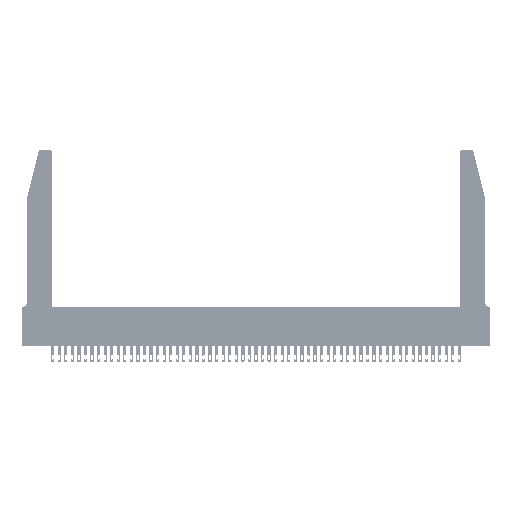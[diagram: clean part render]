
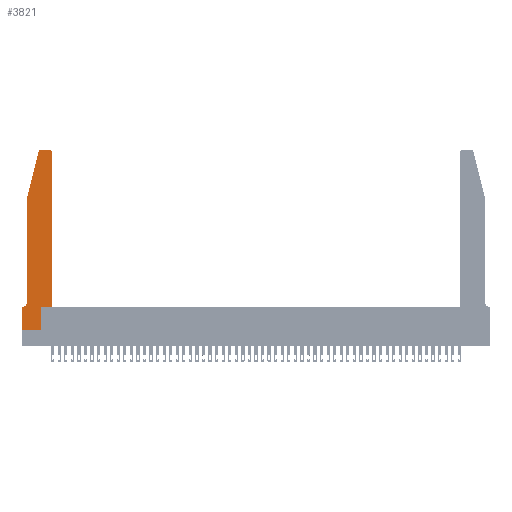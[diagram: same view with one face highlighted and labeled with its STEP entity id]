
A CAD part, top view. The second image highlights one B-rep face of the part: STEP entity #3821.
In plain terms, the highlighted planar face has unit normal (0, 0, 1).
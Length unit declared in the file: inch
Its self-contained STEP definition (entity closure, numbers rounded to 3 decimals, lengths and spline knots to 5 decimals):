
#220 = EDGE_CURVE ( 'NONE', #26783, #27780, #22821, .T. ) ;
#998 = CARTESIAN_POINT ( 'NONE',  ( 0.4505, 0.35, 0.37 ) ) ;
#1057 = EDGE_CURVE ( 'NONE', #46100, #28939, #23431, .T. ) ;
#1085 = VERTEX_POINT ( 'NONE', #23866 ) ;
#2592 = CARTESIAN_POINT ( 'NONE',  ( 0., 0.35, 0.37 ) ) ;
#3109 = DIRECTION ( 'NONE',  ( -0.239, -0.971, 0. ) ) ;
#3821 = ADVANCED_FACE ( 'NONE', ( #13299 ), #21908, .T. ) ;
#4509 = EDGE_CURVE ( 'NONE', #28374, #39760, #44208, .T. ) ;
#4977 = DIRECTION ( 'NONE',  ( 0., 1., 0. ) ) ;
#5112 = VERTEX_POINT ( 'NONE', #32635 ) ;
#6354 = VERTEX_POINT ( 'NONE', #34230 ) ;
#6897 = EDGE_CURVE ( 'NONE', #25672, #26783, #39612, .T. ) ;
#7028 = EDGE_CURVE ( 'NONE', #1085, #46100, #27404, .T. ) ;
#7814 = DIRECTION ( 'NONE',  ( 0., -1., 0. ) ) ;
#8128 = DIRECTION ( 'NONE',  ( -1., 0., 0. ) ) ;
#8252 = ORIENTED_EDGE ( 'NONE', *, *, #4509, .T. ) ;
#8278 = CARTESIAN_POINT ( 'NONE',  ( 0.0755, 2., 0.37 ) ) ;
#10289 = CARTESIAN_POINT ( 'NONE',  ( 0., 0.35, 0.37 ) ) ;
#10340 = CARTESIAN_POINT ( 'NONE',  ( 0.2865, 0.35, 0.37 ) ) ;
#10620 = CARTESIAN_POINT ( 'NONE',  ( 0.0755, 0.42, 0.37 ) ) ;
#12246 = CARTESIAN_POINT ( 'NONE',  ( 0.0055, 0.42, 0.37 ) ) ;
#12318 = CARTESIAN_POINT ( 'NONE',  ( 0.4205, 2.72, 0.37 ) ) ;
#12788 = VECTOR ( 'NONE', #3109, 39.37008 ) ;
#13299 = FACE_OUTER_BOUND ( 'NONE', #31462, .T. ) ;
#14311 = DIRECTION ( 'NONE',  ( -1., 0., 0. ) ) ;
#16272 = DIRECTION ( 'NONE',  ( 0., 0., 1. ) ) ;
#16526 = VECTOR ( 'NONE', #48999, 39.37008 ) ;
#16605 = CARTESIAN_POINT ( 'NONE',  ( 0., 0., 0.37 ) ) ;
#16889 = VECTOR ( 'NONE', #35696, 39.37008 ) ;
#18139 = ORIENTED_EDGE ( 'NONE', *, *, #7028, .T. ) ;
#18206 = ORIENTED_EDGE ( 'NONE', *, *, #23813, .T. ) ;
#18840 = CARTESIAN_POINT ( 'NONE',  ( 0.25487, 2.72718, 0.37 ) ) ;
#19865 = EDGE_CURVE ( 'NONE', #34818, #1085, #37081, .T. ) ;
#20961 = ORIENTED_EDGE ( 'NONE', *, *, #220, .T. ) ;
#21037 = DIRECTION ( 'NONE',  ( 1., 0., 0. ) ) ;
#21895 = AXIS2_PLACEMENT_3D ( 'NONE', #12318, #36790, #21037 ) ;
#21908 = PLANE ( 'NONE',  #37344 ) ;
#22610 = DIRECTION ( 'NONE',  ( 0., -1., 0. ) ) ;
#22821 = LINE ( 'NONE', #25040, #16526 ) ;
#23431 = CIRCLE ( 'NONE', #32250, 0.03 ) ;
#23733 = CARTESIAN_POINT ( 'NONE',  ( 0.0055, 0.35, 0.37 ) ) ;
#23813 = EDGE_CURVE ( 'NONE', #27780, #5112, #41073, .T. ) ;
#23866 = CARTESIAN_POINT ( 'NONE',  ( 0.4205, 2.75, 0.37 ) ) ;
#24027 = CARTESIAN_POINT ( 'NONE',  ( 0.284, 2.72, 0.37 ) ) ;
#24239 = ORIENTED_EDGE ( 'NONE', *, *, #48163, .T. ) ;
#25040 = CARTESIAN_POINT ( 'NONE',  ( 0., 0., 0.37 ) ) ;
#25184 = LINE ( 'NONE', #38951, #12788 ) ;
#25672 = VERTEX_POINT ( 'NONE', #2592 ) ;
#25901 = DIRECTION ( 'NONE',  ( 0., 1., 0. ) ) ;
#26783 = VERTEX_POINT ( 'NONE', #16605 ) ;
#26892 = DIRECTION ( 'NONE',  ( 0., 0., 1. ) ) ;
#27404 = LINE ( 'NONE', #34064, #41087 ) ;
#27405 = LINE ( 'NONE', #31038, #16889 ) ;
#27780 = VERTEX_POINT ( 'NONE', #39206 ) ;
#28033 = DIRECTION ( 'NONE',  ( 1., 0., 0. ) ) ;
#28374 = VERTEX_POINT ( 'NONE', #8278 ) ;
#28939 = VERTEX_POINT ( 'NONE', #18840 ) ;
#29830 = CIRCLE ( 'NONE', #51229, 0.07 ) ;
#30172 = DIRECTION ( 'NONE',  ( 1., 0., 0. ) ) ;
#30941 = VECTOR ( 'NONE', #22610, 39.37008 ) ;
#31038 = CARTESIAN_POINT ( 'NONE',  ( 0.0755, 0.35, 0.37 ) ) ;
#31462 = EDGE_LOOP ( 'NONE', ( #18139, #47641, #24239, #8252, #48288, #35584, #42317, #20961, #18206, #38829, #38232, #39391 ) ) ;
#32250 = AXIS2_PLACEMENT_3D ( 'NONE', #24027, #16272, #28033 ) ;
#32542 = VECTOR ( 'NONE', #4977, 39.37008 ) ;
#32635 = CARTESIAN_POINT ( 'NONE',  ( 0.2865, 0.35, 0.37 ) ) ;
#32901 = CARTESIAN_POINT ( 'NONE',  ( 0., 0., 0.37 ) ) ;
#34064 = CARTESIAN_POINT ( 'NONE',  ( 0.2605, 2.75, 0.37 ) ) ;
#34230 = CARTESIAN_POINT ( 'NONE',  ( 0.4505, 0.35, 0.37 ) ) ;
#34818 = VERTEX_POINT ( 'NONE', #42588 ) ;
#35173 = CARTESIAN_POINT ( 'NONE',  ( 0.284, 2.75, 0.37 ) ) ;
#35584 = ORIENTED_EDGE ( 'NONE', *, *, #49959, .T. ) ;
#35696 = DIRECTION ( 'NONE',  ( -1., 0., 0. ) ) ;
#36790 = DIRECTION ( 'NONE',  ( 0., 0., 1. ) ) ;
#37081 = CIRCLE ( 'NONE', #21895, 0.03 ) ;
#37215 = VERTEX_POINT ( 'NONE', #23733 ) ;
#37344 = AXIS2_PLACEMENT_3D ( 'NONE', #10289, #26892, #30172 ) ;
#38232 = ORIENTED_EDGE ( 'NONE', *, *, #48952, .T. ) ;
#38829 = ORIENTED_EDGE ( 'NONE', *, *, #48463, .T. ) ;
#38951 = CARTESIAN_POINT ( 'NONE',  ( 0.0755, 2., 0.37 ) ) ;
#39206 = CARTESIAN_POINT ( 'NONE',  ( 0.2865, 0., 0.37 ) ) ;
#39391 = ORIENTED_EDGE ( 'NONE', *, *, #19865, .T. ) ;
#39612 = LINE ( 'NONE', #32901, #30941 ) ;
#39760 = VERTEX_POINT ( 'NONE', #10620 ) ;
#39984 = DIRECTION ( 'NONE',  ( 0., 0., -1. ) ) ;
#41073 = LINE ( 'NONE', #10340, #50370 ) ;
#41087 = VECTOR ( 'NONE', #14311, 39.37008 ) ;
#41505 = CARTESIAN_POINT ( 'NONE',  ( 0.4505, 0.35, 0.37 ) ) ;
#42317 = ORIENTED_EDGE ( 'NONE', *, *, #6897, .T. ) ;
#42461 = EDGE_CURVE ( 'NONE', #39760, #37215, #29830, .T. ) ;
#42588 = CARTESIAN_POINT ( 'NONE',  ( 0.4505, 2.72, 0.37 ) ) ;
#43116 = LINE ( 'NONE', #998, #32542 ) ;
#43498 = CARTESIAN_POINT ( 'NONE',  ( 0.0755, 2., 0.37 ) ) ;
#44208 = LINE ( 'NONE', #43498, #47944 ) ;
#45125 = DIRECTION ( 'NONE',  ( 1., 0., 0. ) ) ;
#45662 = LINE ( 'NONE', #41505, #49987 ) ;
#46100 = VERTEX_POINT ( 'NONE', #35173 ) ;
#47641 = ORIENTED_EDGE ( 'NONE', *, *, #1057, .T. ) ;
#47944 = VECTOR ( 'NONE', #7814, 39.37008 ) ;
#48163 = EDGE_CURVE ( 'NONE', #28939, #28374, #25184, .T. ) ;
#48288 = ORIENTED_EDGE ( 'NONE', *, *, #42461, .T. ) ;
#48463 = EDGE_CURVE ( 'NONE', #5112, #6354, #45662, .T. ) ;
#48952 = EDGE_CURVE ( 'NONE', #6354, #34818, #43116, .T. ) ;
#48999 = DIRECTION ( 'NONE',  ( 1., 0., 0. ) ) ;
#49959 = EDGE_CURVE ( 'NONE', #37215, #25672, #27405, .T. ) ;
#49987 = VECTOR ( 'NONE', #45125, 39.37008 ) ;
#50370 = VECTOR ( 'NONE', #25901, 39.37008 ) ;
#51229 = AXIS2_PLACEMENT_3D ( 'NONE', #12246, #39984, #8128 ) ;
